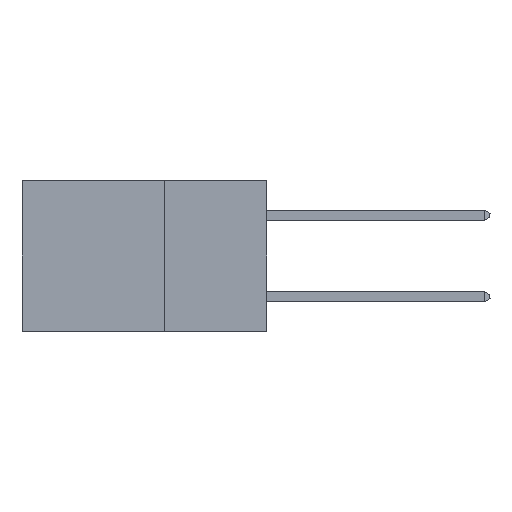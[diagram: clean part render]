
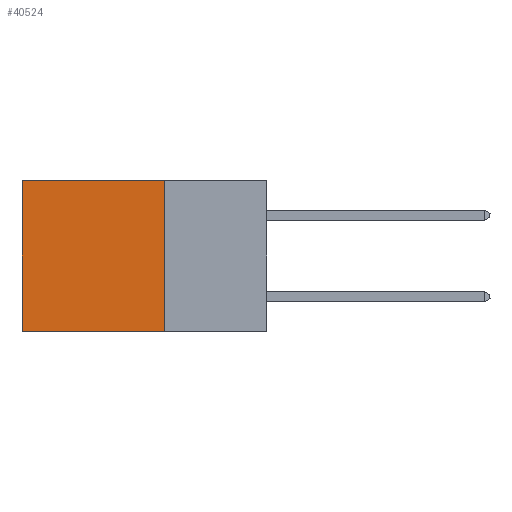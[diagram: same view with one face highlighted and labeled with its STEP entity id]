
A CAD part, left-side view. The second image highlights one B-rep face of the part: STEP entity #40524.
In plain terms, the highlighted planar face has unit normal (-1, 0, 0).
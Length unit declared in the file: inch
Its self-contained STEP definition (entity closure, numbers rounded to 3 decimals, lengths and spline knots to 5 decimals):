
#3586 = CARTESIAN_POINT ( 'NONE',  ( 0.2875, 0.25, 0. ) ) ;
#4118 = CARTESIAN_POINT ( 'NONE',  ( 0.2875, 0.25, 0. ) ) ;
#7676 = EDGE_CURVE ( 'NONE', #32807, #39440, #44830, .T. ) ;
#8692 = CARTESIAN_POINT ( 'NONE',  ( 0.2875, 0.25, 0. ) ) ;
#11089 = ORIENTED_EDGE ( 'NONE', *, *, #17024, .T. ) ;
#12576 = CARTESIAN_POINT ( 'NONE',  ( 0.2875, 0.25, -0.37 ) ) ;
#13612 = LINE ( 'NONE', #46671, #19932 ) ;
#14666 = DIRECTION ( 'NONE',  ( 0., 0., -1. ) ) ;
#14688 = EDGE_CURVE ( 'NONE', #33078, #32807, #38492, .T. ) ;
#17024 = EDGE_CURVE ( 'NONE', #33078, #33749, #29303, .T. ) ;
#19932 = VECTOR ( 'NONE', #46520, 39.37008 ) ;
#21980 = ORIENTED_EDGE ( 'NONE', *, *, #14688, .F. ) ;
#23989 = CARTESIAN_POINT ( 'NONE',  ( 0.2875, 0.6, -0.37 ) ) ;
#28060 = FACE_OUTER_BOUND ( 'NONE', #35409, .T. ) ;
#29303 = LINE ( 'NONE', #8692, #40190 ) ;
#29673 = CARTESIAN_POINT ( 'NONE',  ( 0.2875, 0.6, 0. ) ) ;
#30109 = AXIS2_PLACEMENT_3D ( 'NONE', #4118, #36727, #14666 ) ;
#31300 = DIRECTION ( 'NONE',  ( 0., 0., -1. ) ) ;
#32807 = VERTEX_POINT ( 'NONE', #12576 ) ;
#33078 = VERTEX_POINT ( 'NONE', #3586 ) ;
#33204 = PLANE ( 'NONE',  #30109 ) ;
#33749 = VERTEX_POINT ( 'NONE', #29673 ) ;
#33906 = VECTOR ( 'NONE', #31300, 39.37008 ) ;
#34131 = ORIENTED_EDGE ( 'NONE', *, *, #46801, .T. ) ;
#35409 = EDGE_LOOP ( 'NONE', ( #34131, #36232, #21980, #11089 ) ) ;
#36232 = ORIENTED_EDGE ( 'NONE', *, *, #7676, .F. ) ;
#36266 = VECTOR ( 'NONE', #41690, 39.37008 ) ;
#36727 = DIRECTION ( 'NONE',  ( 1., 0., 0. ) ) ;
#37892 = CARTESIAN_POINT ( 'NONE',  ( 0.2875, 0.25, -0.37 ) ) ;
#37957 = DIRECTION ( 'NONE',  ( 0., 1., 0. ) ) ;
#38492 = LINE ( 'NONE', #42484, #33906 ) ;
#39440 = VERTEX_POINT ( 'NONE', #23989 ) ;
#40190 = VECTOR ( 'NONE', #37957, 39.37008 ) ;
#40524 = ADVANCED_FACE ( 'NONE', ( #28060 ), #33204, .F. ) ;
#41690 = DIRECTION ( 'NONE',  ( 0., 1., 0. ) ) ;
#42484 = CARTESIAN_POINT ( 'NONE',  ( 0.2875, 0.25, 0. ) ) ;
#44830 = LINE ( 'NONE', #37892, #36266 ) ;
#46520 = DIRECTION ( 'NONE',  ( 0., 0., -1. ) ) ;
#46671 = CARTESIAN_POINT ( 'NONE',  ( 0.2875, 0.6, 0. ) ) ;
#46801 = EDGE_CURVE ( 'NONE', #33749, #39440, #13612, .T. ) ;
